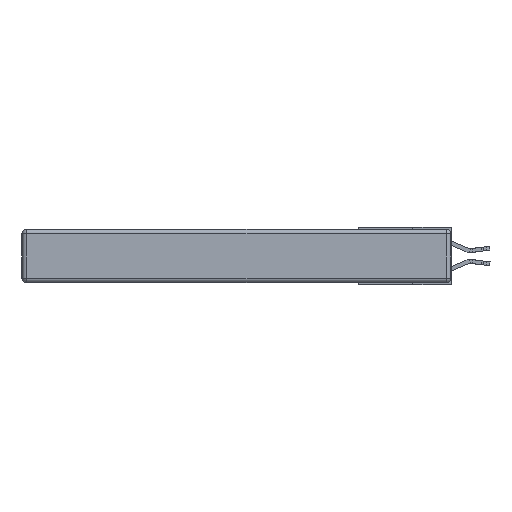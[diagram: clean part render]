
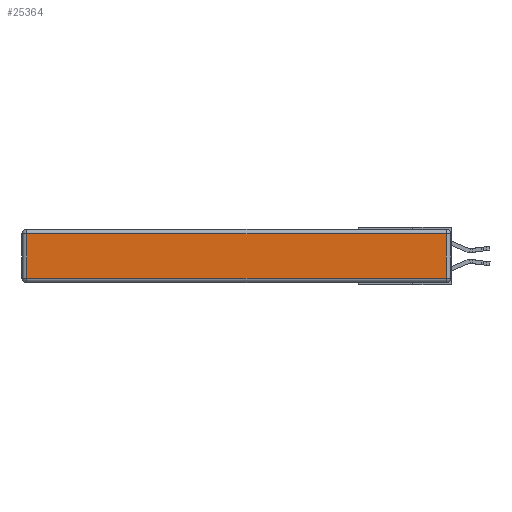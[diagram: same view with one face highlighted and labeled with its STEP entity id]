
A CAD part, left-side view. The second image highlights one B-rep face of the part: STEP entity #25364.
In plain terms, the highlighted planar face has unit normal (-1, 0, 0).
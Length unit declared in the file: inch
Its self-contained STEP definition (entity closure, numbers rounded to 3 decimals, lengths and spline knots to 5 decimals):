
#2347 = ORIENTED_EDGE ( 'NONE', *, *, #6746, .T. ) ;
#3731 = VERTEX_POINT ( 'NONE', #27505 ) ;
#5088 = EDGE_CURVE ( 'NONE', #8858, #29792, #18435, .T. ) ;
#6122 = VECTOR ( 'NONE', #7013, 39.37008 ) ;
#6382 = DIRECTION ( 'NONE',  ( 0., 0., -1. ) ) ;
#6746 = EDGE_CURVE ( 'NONE', #3731, #10480, #21026, .T. ) ;
#6881 = DIRECTION ( 'NONE',  ( -1., 0., 0. ) ) ;
#6889 = ORIENTED_EDGE ( 'NONE', *, *, #5088, .T. ) ;
#7013 = DIRECTION ( 'NONE',  ( 0., 0., 1. ) ) ;
#7948 = VECTOR ( 'NONE', #6382, 39.37008 ) ;
#8858 = VERTEX_POINT ( 'NONE', #11535 ) ;
#10480 = VERTEX_POINT ( 'NONE', #27637 ) ;
#11069 = CARTESIAN_POINT ( 'NONE',  ( 0., 2.72, -0.343 ) ) ;
#11535 = CARTESIAN_POINT ( 'NONE',  ( 0., 2.72, -0.313 ) ) ;
#12134 = VECTOR ( 'NONE', #20724, 39.37008 ) ;
#13860 = ORIENTED_EDGE ( 'NONE', *, *, #27345, .T. ) ;
#14186 = FACE_OUTER_BOUND ( 'NONE', #21147, .T. ) ;
#14259 = DIRECTION ( 'NONE',  ( 0., 0., 1. ) ) ;
#15271 = DIRECTION ( 'NONE',  ( 0., -1., 0. ) ) ;
#18435 = LINE ( 'NONE', #22693, #18812 ) ;
#18812 = VECTOR ( 'NONE', #15271, 39.37008 ) ;
#19203 = ORIENTED_EDGE ( 'NONE', *, *, #20310, .T. ) ;
#20310 = EDGE_CURVE ( 'NONE', #29792, #3731, #23746, .T. ) ;
#20724 = DIRECTION ( 'NONE',  ( 0., 1., 0. ) ) ;
#21026 = LINE ( 'NONE', #23155, #12134 ) ;
#21147 = EDGE_LOOP ( 'NONE', ( #6889, #19203, #2347, #13860 ) ) ;
#22693 = CARTESIAN_POINT ( 'NONE',  ( 0., 0., -0.313 ) ) ;
#23155 = CARTESIAN_POINT ( 'NONE',  ( 0., 2.75, -0.03 ) ) ;
#23532 = AXIS2_PLACEMENT_3D ( 'NONE', #31552, #6881, #14259 ) ;
#23746 = LINE ( 'NONE', #24389, #6122 ) ;
#24389 = CARTESIAN_POINT ( 'NONE',  ( 0., 0.03, -0.343 ) ) ;
#25364 = ADVANCED_FACE ( 'NONE', ( #14186 ), #31344, .T. ) ;
#26414 = LINE ( 'NONE', #11069, #7948 ) ;
#27345 = EDGE_CURVE ( 'NONE', #10480, #8858, #26414, .T. ) ;
#27505 = CARTESIAN_POINT ( 'NONE',  ( 0., 0.03, -0.03 ) ) ;
#27637 = CARTESIAN_POINT ( 'NONE',  ( 0., 2.72, -0.03 ) ) ;
#29792 = VERTEX_POINT ( 'NONE', #30438 ) ;
#30438 = CARTESIAN_POINT ( 'NONE',  ( 0., 0.03, -0.313 ) ) ;
#31344 = PLANE ( 'NONE',  #23532 ) ;
#31552 = CARTESIAN_POINT ( 'NONE',  ( 0., 0., -0.343 ) ) ;
